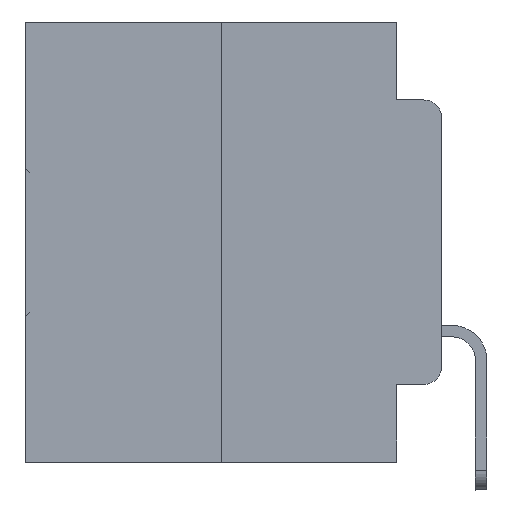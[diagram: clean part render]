
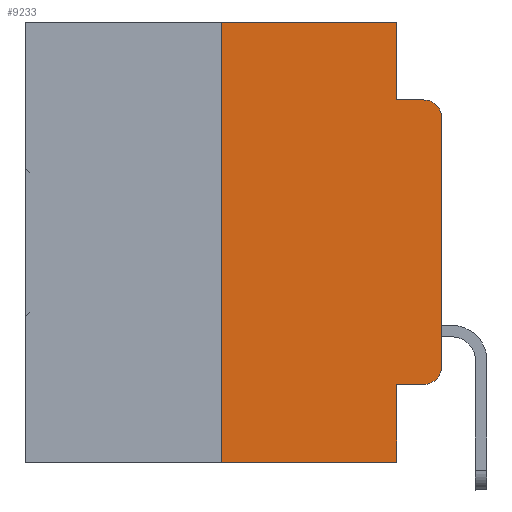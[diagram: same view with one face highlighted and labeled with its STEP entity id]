
A CAD part, left-side view. The second image highlights one B-rep face of the part: STEP entity #9233.
In plain terms, the highlighted planar face has unit normal (-1, 0, 0).
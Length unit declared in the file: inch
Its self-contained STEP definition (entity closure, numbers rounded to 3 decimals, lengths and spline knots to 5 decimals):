
#41 = DIRECTION ( 'NONE',  ( 0., 0., -1. ) ) ;
#85 = CIRCLE ( 'NONE', #10297, 0.02 ) ;
#250 = VERTEX_POINT ( 'NONE', #16692 ) ;
#773 = AXIS2_PLACEMENT_3D ( 'NONE', #30283, #5860, #15653 ) ;
#1105 = LINE ( 'NONE', #18258, #9975 ) ;
#1328 = VERTEX_POINT ( 'NONE', #27809 ) ;
#1462 = CARTESIAN_POINT ( 'NONE',  ( 0., 0.473, -0.5 ) ) ;
#1548 = LINE ( 'NONE', #25771, #16226 ) ;
#2281 = CARTESIAN_POINT ( 'NONE',  ( 0., 0.02, -0.1085 ) ) ;
#2592 = ORIENTED_EDGE ( 'NONE', *, *, #11623, .T. ) ;
#2904 = EDGE_CURVE ( 'NONE', #1328, #250, #14564, .T. ) ;
#3852 = VERTEX_POINT ( 'NONE', #30383 ) ;
#4222 = VECTOR ( 'NONE', #23192, 39.37008 ) ;
#4585 = VERTEX_POINT ( 'NONE', #14535 ) ;
#4880 = ORIENTED_EDGE ( 'NONE', *, *, #8930, .F. ) ;
#5179 = DIRECTION ( 'NONE',  ( 0., 0., -1. ) ) ;
#5850 = CARTESIAN_POINT ( 'NONE',  ( 0., 0.25, 0. ) ) ;
#5860 = DIRECTION ( 'NONE',  ( 1., 0., 0. ) ) ;
#7035 = EDGE_CURVE ( 'NONE', #250, #25867, #12045, .T. ) ;
#7239 = DIRECTION ( 'NONE',  ( -1., 0., 0. ) ) ;
#7353 = EDGE_CURVE ( 'NONE', #21036, #27652, #23444, .T. ) ;
#7677 = CARTESIAN_POINT ( 'NONE',  ( 0., 0.051, -0.4115 ) ) ;
#8705 = CARTESIAN_POINT ( 'NONE',  ( 0., 0., -0.1085 ) ) ;
#8930 = EDGE_CURVE ( 'NONE', #22568, #27652, #1105, .T. ) ;
#9159 = VECTOR ( 'NONE', #22277, 39.37008 ) ;
#9233 = ADVANCED_FACE ( 'NONE', ( #20948 ), #30435, .F. ) ;
#9640 = DIRECTION ( 'NONE',  ( 0., 0., -1. ) ) ;
#9890 = VECTOR ( 'NONE', #12169, 39.37008 ) ;
#9975 = VECTOR ( 'NONE', #28232, 39.37008 ) ;
#10297 = AXIS2_PLACEMENT_3D ( 'NONE', #27778, #20855, #5179 ) ;
#11005 = EDGE_CURVE ( 'NONE', #4585, #31068, #13559, .T. ) ;
#11623 = EDGE_CURVE ( 'NONE', #31068, #31606, #13659, .T. ) ;
#12045 = LINE ( 'NONE', #24417, #13503 ) ;
#12169 = DIRECTION ( 'NONE',  ( 0., -1., 0. ) ) ;
#12287 = EDGE_CURVE ( 'NONE', #22568, #3852, #1548, .T. ) ;
#13254 = CARTESIAN_POINT ( 'NONE',  ( 0., 0., 0. ) ) ;
#13503 = VECTOR ( 'NONE', #9640, 39.37008 ) ;
#13559 = LINE ( 'NONE', #13254, #23439 ) ;
#13622 = ORIENTED_EDGE ( 'NONE', *, *, #11005, .T. ) ;
#13659 = CIRCLE ( 'NONE', #21868, 0.02 ) ;
#14535 = CARTESIAN_POINT ( 'NONE',  ( 0., 0., -0.3915 ) ) ;
#14564 = LINE ( 'NONE', #16982, #9159 ) ;
#14707 = CARTESIAN_POINT ( 'NONE',  ( 0., 0.25, -0.5 ) ) ;
#15653 = DIRECTION ( 'NONE',  ( 0., 0., -1. ) ) ;
#15660 = DIRECTION ( 'NONE',  ( 0., -1., 0. ) ) ;
#15733 = ORIENTED_EDGE ( 'NONE', *, *, #7035, .F. ) ;
#15809 = CARTESIAN_POINT ( 'NONE',  ( 0., 0.051, -0.0885 ) ) ;
#15957 = ORIENTED_EDGE ( 'NONE', *, *, #16572, .T. ) ;
#16226 = VECTOR ( 'NONE', #15660, 39.37008 ) ;
#16572 = EDGE_CURVE ( 'NONE', #3852, #4585, #85, .T. ) ;
#16692 = CARTESIAN_POINT ( 'NONE',  ( 0., 0.051, 0. ) ) ;
#16982 = CARTESIAN_POINT ( 'NONE',  ( 0., 0.473, 0. ) ) ;
#18051 = LINE ( 'NONE', #5850, #21296 ) ;
#18258 = CARTESIAN_POINT ( 'NONE',  ( 0., 0.051, 0. ) ) ;
#18625 = CARTESIAN_POINT ( 'NONE',  ( 0., 0.051, -0.5 ) ) ;
#20453 = LINE ( 'NONE', #15809, #4222 ) ;
#20792 = ORIENTED_EDGE ( 'NONE', *, *, #7353, .T. ) ;
#20801 = ORIENTED_EDGE ( 'NONE', *, *, #12287, .T. ) ;
#20855 = DIRECTION ( 'NONE',  ( -1., 0., 0. ) ) ;
#20948 = FACE_OUTER_BOUND ( 'NONE', #30002, .T. ) ;
#21036 = VERTEX_POINT ( 'NONE', #14707 ) ;
#21296 = VECTOR ( 'NONE', #23513, 39.37008 ) ;
#21868 = AXIS2_PLACEMENT_3D ( 'NONE', #2281, #7239, #41 ) ;
#22277 = DIRECTION ( 'NONE',  ( 0., -1., 0. ) ) ;
#22568 = VERTEX_POINT ( 'NONE', #7677 ) ;
#23050 = DIRECTION ( 'NONE',  ( 0., 0., 1. ) ) ;
#23192 = DIRECTION ( 'NONE',  ( 0., -1., 0. ) ) ;
#23285 = ORIENTED_EDGE ( 'NONE', *, *, #28799, .F. ) ;
#23439 = VECTOR ( 'NONE', #23050, 39.37008 ) ;
#23444 = LINE ( 'NONE', #1462, #9890 ) ;
#23513 = DIRECTION ( 'NONE',  ( 0., 0., 1. ) ) ;
#23768 = CARTESIAN_POINT ( 'NONE',  ( 0., 0.02, -0.0885 ) ) ;
#24212 = CARTESIAN_POINT ( 'NONE',  ( 0., 0.051, -0.0885 ) ) ;
#24417 = CARTESIAN_POINT ( 'NONE',  ( 0., 0.051, 0. ) ) ;
#25771 = CARTESIAN_POINT ( 'NONE',  ( 0., 0.051, -0.4115 ) ) ;
#25867 = VERTEX_POINT ( 'NONE', #24212 ) ;
#27652 = VERTEX_POINT ( 'NONE', #18625 ) ;
#27778 = CARTESIAN_POINT ( 'NONE',  ( 0., 0.02, -0.3915 ) ) ;
#27809 = CARTESIAN_POINT ( 'NONE',  ( 0., 0.25, 0. ) ) ;
#28232 = DIRECTION ( 'NONE',  ( 0., 0., -1. ) ) ;
#28799 = EDGE_CURVE ( 'NONE', #25867, #31606, #20453, .T. ) ;
#29718 = ORIENTED_EDGE ( 'NONE', *, *, #30132, .F. ) ;
#30002 = EDGE_LOOP ( 'NONE', ( #13622, #2592, #23285, #15733, #31009, #29718, #20792, #4880, #20801, #15957 ) ) ;
#30132 = EDGE_CURVE ( 'NONE', #21036, #1328, #18051, .T. ) ;
#30283 = CARTESIAN_POINT ( 'NONE',  ( 0., 0.473, 0. ) ) ;
#30383 = CARTESIAN_POINT ( 'NONE',  ( 0., 0.02, -0.4115 ) ) ;
#30435 = PLANE ( 'NONE',  #773 ) ;
#31009 = ORIENTED_EDGE ( 'NONE', *, *, #2904, .F. ) ;
#31068 = VERTEX_POINT ( 'NONE', #8705 ) ;
#31606 = VERTEX_POINT ( 'NONE', #23768 ) ;
